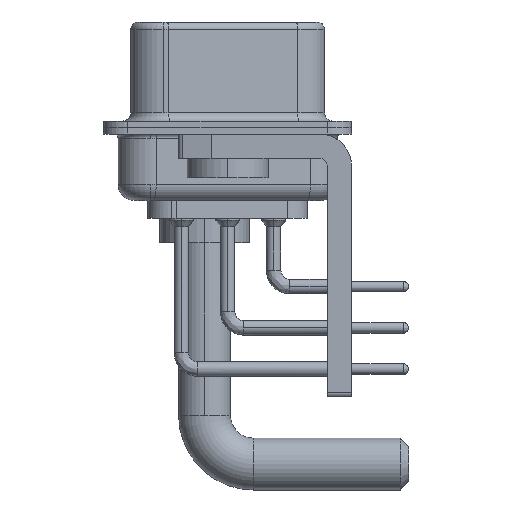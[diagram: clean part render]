
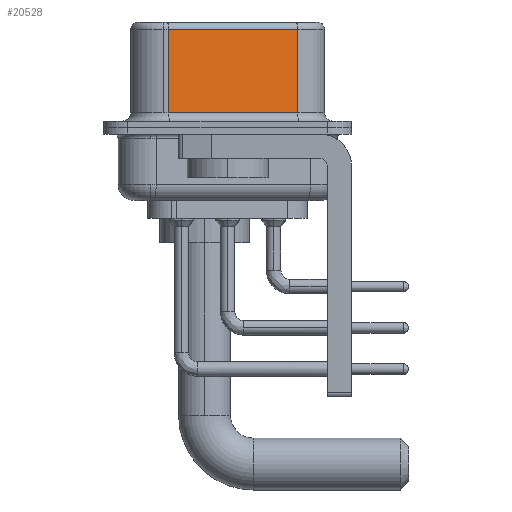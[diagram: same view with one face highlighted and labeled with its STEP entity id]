
A CAD part, left-side view. The second image highlights one B-rep face of the part: STEP entity #20528.
In plain terms, the highlighted planar face has unit normal (-0.985, -0.174, 0).
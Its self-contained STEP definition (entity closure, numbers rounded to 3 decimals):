
#1090 = EDGE_LOOP ( 'NONE', ( #18684, #7425, #20769, #9899 ) ) ;
#3385 = DIRECTION ( 'NONE',  ( -0.174, 0.985, 0. ) ) ;
#5447 = VECTOR ( 'NONE', #28664, 1000. ) ;
#6027 = CARTESIAN_POINT ( 'NONE',  ( 5.132, -4.322, 6.02 ) ) ;
#6210 = LINE ( 'NONE', #6027, #17552 ) ;
#7261 = LINE ( 'NONE', #10083, #22344 ) ;
#7425 = ORIENTED_EDGE ( 'NONE', *, *, #37005, .T. ) ;
#9634 = CARTESIAN_POINT ( 'NONE',  ( 3.73, 3.628, 0.9 ) ) ;
#9899 = ORIENTED_EDGE ( 'NONE', *, *, #35019, .T. ) ;
#10083 = CARTESIAN_POINT ( 'NONE',  ( 5.132, -4.322, 6.52 ) ) ;
#12931 = CARTESIAN_POINT ( 'NONE',  ( 3.73, 3.628, 6.52 ) ) ;
#14081 = PLANE ( 'NONE',  #15341 ) ;
#15001 = EDGE_CURVE ( 'NONE', #17053, #16285, #7261, .T. ) ;
#15341 = AXIS2_PLACEMENT_3D ( 'NONE', #19712, #22537, #28165 ) ;
#16285 = VERTEX_POINT ( 'NONE', #36515 ) ;
#17053 = VERTEX_POINT ( 'NONE', #27560 ) ;
#17552 = VECTOR ( 'NONE', #3385, 1000. ) ;
#18684 = ORIENTED_EDGE ( 'NONE', *, *, #15001, .F. ) ;
#18879 = VERTEX_POINT ( 'NONE', #36574 ) ;
#19712 = CARTESIAN_POINT ( 'NONE',  ( 5.132, -4.322, 6.52 ) ) ;
#20207 = LINE ( 'NONE', #23032, #5447 ) ;
#20528 = ADVANCED_FACE ( 'NONE', ( #25532 ), #14081, .F. ) ;
#20769 = ORIENTED_EDGE ( 'NONE', *, *, #24653, .T. ) ;
#22344 = VECTOR ( 'NONE', #24741, 1000. ) ;
#22537 = DIRECTION ( 'NONE',  ( 0.985, 0.174, 0. ) ) ;
#23032 = CARTESIAN_POINT ( 'NONE',  ( 5.132, -4.322, 0.9 ) ) ;
#24653 = EDGE_CURVE ( 'NONE', #18879, #36797, #27222, .T. ) ;
#24741 = DIRECTION ( 'NONE',  ( 0., 0., -1. ) ) ;
#25532 = FACE_OUTER_BOUND ( 'NONE', #1090, .T. ) ;
#27222 = LINE ( 'NONE', #12931, #29305 ) ;
#27560 = CARTESIAN_POINT ( 'NONE',  ( 5.132, -4.322, 6.02 ) ) ;
#28165 = DIRECTION ( 'NONE',  ( -0.174, 0.985, 0. ) ) ;
#28664 = DIRECTION ( 'NONE',  ( 0.174, -0.985, 0. ) ) ;
#29305 = VECTOR ( 'NONE', #32120, 1000. ) ;
#32120 = DIRECTION ( 'NONE',  ( 0., 0., -1. ) ) ;
#35019 = EDGE_CURVE ( 'NONE', #36797, #16285, #20207, .T. ) ;
#36515 = CARTESIAN_POINT ( 'NONE',  ( 5.132, -4.322, 0.9 ) ) ;
#36574 = CARTESIAN_POINT ( 'NONE',  ( 3.73, 3.628, 6.02 ) ) ;
#36797 = VERTEX_POINT ( 'NONE', #9634 ) ;
#37005 = EDGE_CURVE ( 'NONE', #17053, #18879, #6210, .T. ) ;
